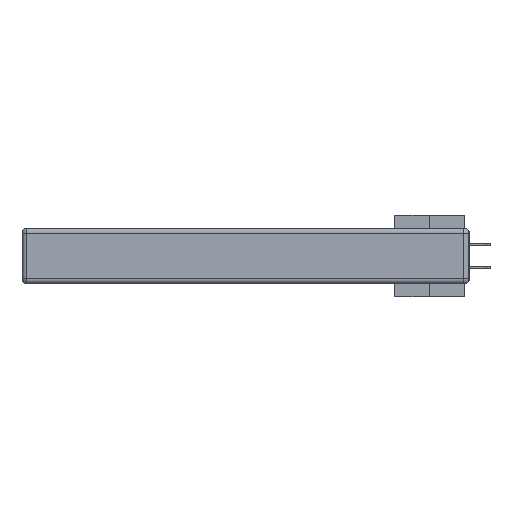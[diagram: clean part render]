
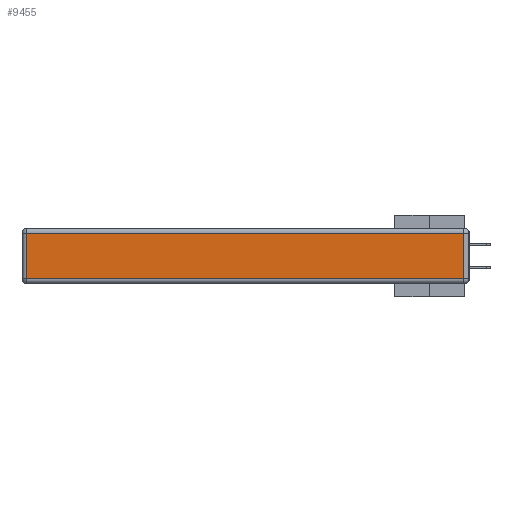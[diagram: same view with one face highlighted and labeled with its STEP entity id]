
A CAD part, left-side view. The second image highlights one B-rep face of the part: STEP entity #9455.
In plain terms, the highlighted planar face has unit normal (-1, 0, 0).
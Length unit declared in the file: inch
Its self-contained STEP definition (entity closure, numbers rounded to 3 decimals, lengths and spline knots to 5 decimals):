
#9443 = CARTESIAN_POINT ( 'NONE',  ( 0., 2.75, -0.03 ) ) ;
#9455 = ADVANCED_FACE ( 'NONE', ( #32361 ), #21143, .T. ) ;
#10141 = EDGE_CURVE ( 'NONE', #39887, #15107, #15600, .T. ) ;
#13106 = CARTESIAN_POINT ( 'NONE',  ( 0., 0.03, -0.03 ) ) ;
#13306 = DIRECTION ( 'NONE',  ( 0., 0., 1. ) ) ;
#14291 = VERTEX_POINT ( 'NONE', #31932 ) ;
#15107 = VERTEX_POINT ( 'NONE', #22538 ) ;
#15504 = EDGE_LOOP ( 'NONE', ( #38576, #32035, #15542, #45136 ) ) ;
#15542 = ORIENTED_EDGE ( 'NONE', *, *, #10141, .T. ) ;
#15600 = LINE ( 'NONE', #9443, #21572 ) ;
#16910 = CARTESIAN_POINT ( 'NONE',  ( 0., 0., -0.313 ) ) ;
#18217 = DIRECTION ( 'NONE',  ( 0., 1., 0. ) ) ;
#19792 = LINE ( 'NONE', #16910, #39957 ) ;
#19946 = VECTOR ( 'NONE', #26552, 39.37008 ) ;
#21143 = PLANE ( 'NONE',  #37462 ) ;
#21572 = VECTOR ( 'NONE', #18217, 39.37008 ) ;
#21709 = EDGE_CURVE ( 'NONE', #15107, #26392, #37147, .T. ) ;
#22538 = CARTESIAN_POINT ( 'NONE',  ( 0., 2.72, -0.03 ) ) ;
#26392 = VERTEX_POINT ( 'NONE', #42958 ) ;
#26552 = DIRECTION ( 'NONE',  ( 0., 0., -1. ) ) ;
#31932 = CARTESIAN_POINT ( 'NONE',  ( 0., 0.03, -0.313 ) ) ;
#32035 = ORIENTED_EDGE ( 'NONE', *, *, #35132, .T. ) ;
#32361 = FACE_OUTER_BOUND ( 'NONE', #15504, .T. ) ;
#32899 = DIRECTION ( 'NONE',  ( -1., 0., 0. ) ) ;
#34160 = CARTESIAN_POINT ( 'NONE',  ( 0., 2.72, -0.343 ) ) ;
#35132 = EDGE_CURVE ( 'NONE', #14291, #39887, #44470, .T. ) ;
#37147 = LINE ( 'NONE', #34160, #19946 ) ;
#37462 = AXIS2_PLACEMENT_3D ( 'NONE', #47467, #32899, #13306 ) ;
#38576 = ORIENTED_EDGE ( 'NONE', *, *, #43236, .T. ) ;
#39887 = VERTEX_POINT ( 'NONE', #13106 ) ;
#39957 = VECTOR ( 'NONE', #46933, 39.37008 ) ;
#42958 = CARTESIAN_POINT ( 'NONE',  ( 0., 2.72, -0.313 ) ) ;
#43236 = EDGE_CURVE ( 'NONE', #26392, #14291, #19792, .T. ) ;
#44470 = LINE ( 'NONE', #45402, #46878 ) ;
#45136 = ORIENTED_EDGE ( 'NONE', *, *, #21709, .T. ) ;
#45402 = CARTESIAN_POINT ( 'NONE',  ( 0., 0.03, -0.343 ) ) ;
#46878 = VECTOR ( 'NONE', #48842, 39.37008 ) ;
#46933 = DIRECTION ( 'NONE',  ( 0., -1., 0. ) ) ;
#47467 = CARTESIAN_POINT ( 'NONE',  ( 0., 0., -0.343 ) ) ;
#48842 = DIRECTION ( 'NONE',  ( 0., 0., 1. ) ) ;
